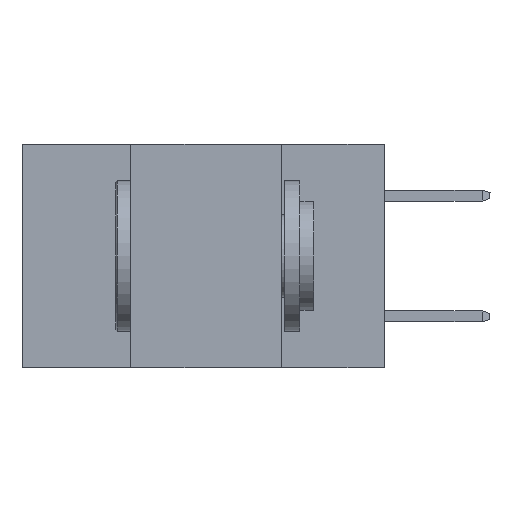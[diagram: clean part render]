
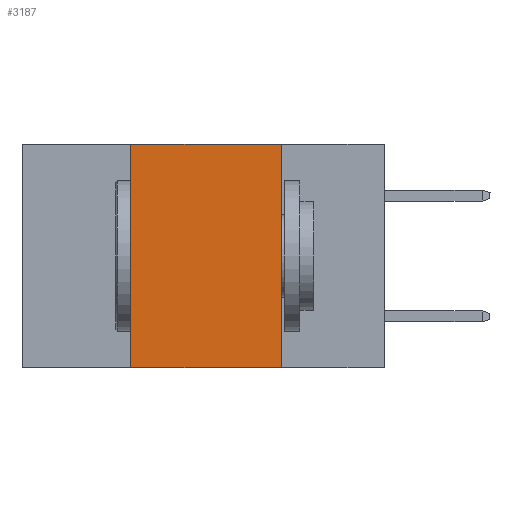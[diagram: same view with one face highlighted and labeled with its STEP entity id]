
A CAD part, left-side view. The second image highlights one B-rep face of the part: STEP entity #3187.
In plain terms, the highlighted planar face has unit normal (-1, 0, 0).
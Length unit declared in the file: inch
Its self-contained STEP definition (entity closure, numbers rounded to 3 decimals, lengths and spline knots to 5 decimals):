
#30 = CARTESIAN_POINT ( 'NONE',  ( 0., 0.17, 0. ) ) ;
#1579 = DIRECTION ( 'NONE',  ( 0., -1., 0. ) ) ;
#2944 = CARTESIAN_POINT ( 'NONE',  ( 0., 0.6, 0. ) ) ;
#3046 = PLANE ( 'NONE',  #17341 ) ;
#3180 = ORIENTED_EDGE ( 'NONE', *, *, #9513, .F. ) ;
#3187 = ADVANCED_FACE ( 'NONE', ( #14093 ), #3046, .F. ) ;
#4734 = CARTESIAN_POINT ( 'NONE',  ( 0., 0.17, -0.37 ) ) ;
#4920 = LINE ( 'NONE', #19586, #22101 ) ;
#5015 = VECTOR ( 'NONE', #1579, 39.37008 ) ;
#5056 = VERTEX_POINT ( 'NONE', #4734 ) ;
#5687 = LINE ( 'NONE', #28321, #5015 ) ;
#9240 = EDGE_LOOP ( 'NONE', ( #13156, #3180, #25311, #17235 ) ) ;
#9513 = EDGE_CURVE ( 'NONE', #9748, #21754, #5687, .T. ) ;
#9748 = VERTEX_POINT ( 'NONE', #16863 ) ;
#13156 = ORIENTED_EDGE ( 'NONE', *, *, #23658, .F. ) ;
#14093 = FACE_OUTER_BOUND ( 'NONE', #9240, .T. ) ;
#15419 = CARTESIAN_POINT ( 'NONE',  ( 0., 0.17, 0. ) ) ;
#15474 = DIRECTION ( 'NONE',  ( 0., 0., -1. ) ) ;
#16571 = DIRECTION ( 'NONE',  ( 1., 0., 0. ) ) ;
#16638 = VERTEX_POINT ( 'NONE', #23774 ) ;
#16863 = CARTESIAN_POINT ( 'NONE',  ( 0., 0.42, 0. ) ) ;
#17235 = ORIENTED_EDGE ( 'NONE', *, *, #23818, .T. ) ;
#17341 = AXIS2_PLACEMENT_3D ( 'NONE', #2944, #16571, #21243 ) ;
#19586 = CARTESIAN_POINT ( 'NONE',  ( 0., 0.42, 0. ) ) ;
#19784 = DIRECTION ( 'NONE',  ( 0., 0., 1. ) ) ;
#20137 = VECTOR ( 'NONE', #27057, 39.37008 ) ;
#21243 = DIRECTION ( 'NONE',  ( 0., 0., -1. ) ) ;
#21754 = VERTEX_POINT ( 'NONE', #15419 ) ;
#22101 = VECTOR ( 'NONE', #19784, 39.37008 ) ;
#22273 = LINE ( 'NONE', #30, #22969 ) ;
#22969 = VECTOR ( 'NONE', #15474, 39.37008 ) ;
#23658 = EDGE_CURVE ( 'NONE', #21754, #5056, #22273, .T. ) ;
#23774 = CARTESIAN_POINT ( 'NONE',  ( 0., 0.42, -0.37 ) ) ;
#23818 = EDGE_CURVE ( 'NONE', #16638, #5056, #26038, .T. ) ;
#24933 = CARTESIAN_POINT ( 'NONE',  ( 0., 0.6, -0.37 ) ) ;
#25311 = ORIENTED_EDGE ( 'NONE', *, *, #26889, .F. ) ;
#26038 = LINE ( 'NONE', #24933, #20137 ) ;
#26889 = EDGE_CURVE ( 'NONE', #16638, #9748, #4920, .T. ) ;
#27057 = DIRECTION ( 'NONE',  ( 0., -1., 0. ) ) ;
#28321 = CARTESIAN_POINT ( 'NONE',  ( 0., 0.6, 0. ) ) ;
